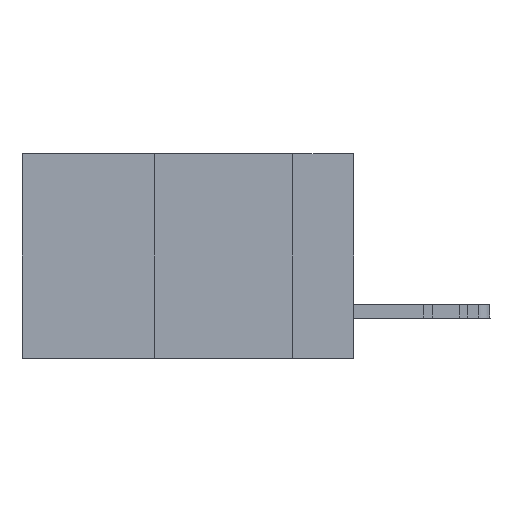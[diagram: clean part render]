
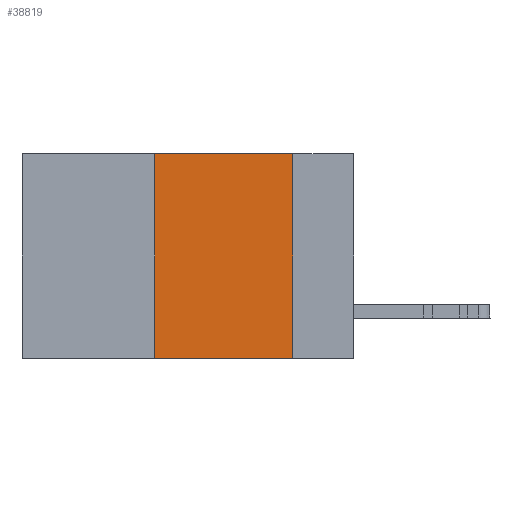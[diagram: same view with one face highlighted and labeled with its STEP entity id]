
A CAD part, left-side view. The second image highlights one B-rep face of the part: STEP entity #38819.
In plain terms, the highlighted planar face has unit normal (-1, 0, 0).
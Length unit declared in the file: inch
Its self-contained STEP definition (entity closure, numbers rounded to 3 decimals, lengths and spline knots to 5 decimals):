
#662 = CARTESIAN_POINT ( 'NONE',  ( 0., 0.36, 0. ) ) ;
#795 = VERTEX_POINT ( 'NONE', #25790 ) ;
#1541 = EDGE_CURVE ( 'NONE', #22153, #28215, #35468, .T. ) ;
#4881 = DIRECTION ( 'NONE',  ( 0., -1., 0. ) ) ;
#6494 = CARTESIAN_POINT ( 'NONE',  ( 0., 0.6, -0.37 ) ) ;
#7381 = VECTOR ( 'NONE', #44340, 39.37008 ) ;
#8488 = EDGE_CURVE ( 'NONE', #34589, #22153, #35099, .T. ) ;
#11538 = VECTOR ( 'NONE', #4881, 39.37008 ) ;
#13458 = CARTESIAN_POINT ( 'NONE',  ( 0., 0.6, 0. ) ) ;
#14044 = CARTESIAN_POINT ( 'NONE',  ( 0., 0.36, 0. ) ) ;
#14778 = DIRECTION ( 'NONE',  ( 0., 0., 1. ) ) ;
#15406 = ORIENTED_EDGE ( 'NONE', *, *, #8488, .F. ) ;
#16712 = LINE ( 'NONE', #23260, #7381 ) ;
#16812 = DIRECTION ( 'NONE',  ( 1., 0., 0. ) ) ;
#17992 = AXIS2_PLACEMENT_3D ( 'NONE', #13458, #16812, #44727 ) ;
#22118 = CARTESIAN_POINT ( 'NONE',  ( 0., 0.36, -0.37 ) ) ;
#22153 = VERTEX_POINT ( 'NONE', #662 ) ;
#23260 = CARTESIAN_POINT ( 'NONE',  ( 0., 0.11, 0. ) ) ;
#24298 = ORIENTED_EDGE ( 'NONE', *, *, #29861, .F. ) ;
#24832 = VECTOR ( 'NONE', #34191, 39.37008 ) ;
#25790 = CARTESIAN_POINT ( 'NONE',  ( 0., 0.11, -0.37 ) ) ;
#26591 = CARTESIAN_POINT ( 'NONE',  ( 0., 0.11, 0. ) ) ;
#28215 = VERTEX_POINT ( 'NONE', #26591 ) ;
#29746 = FACE_OUTER_BOUND ( 'NONE', #33715, .T. ) ;
#29861 = EDGE_CURVE ( 'NONE', #28215, #795, #16712, .T. ) ;
#31331 = ORIENTED_EDGE ( 'NONE', *, *, #1541, .F. ) ;
#33715 = EDGE_LOOP ( 'NONE', ( #24298, #31331, #15406, #44149 ) ) ;
#34191 = DIRECTION ( 'NONE',  ( 0., -1., 0. ) ) ;
#34589 = VERTEX_POINT ( 'NONE', #22118 ) ;
#35099 = LINE ( 'NONE', #14044, #43926 ) ;
#35468 = LINE ( 'NONE', #39779, #11538 ) ;
#37943 = LINE ( 'NONE', #6494, #24832 ) ;
#38147 = EDGE_CURVE ( 'NONE', #34589, #795, #37943, .T. ) ;
#38819 = ADVANCED_FACE ( 'NONE', ( #29746 ), #41371, .F. ) ;
#39779 = CARTESIAN_POINT ( 'NONE',  ( 0., 0.6, 0. ) ) ;
#41371 = PLANE ( 'NONE',  #17992 ) ;
#43926 = VECTOR ( 'NONE', #14778, 39.37008 ) ;
#44149 = ORIENTED_EDGE ( 'NONE', *, *, #38147, .T. ) ;
#44340 = DIRECTION ( 'NONE',  ( 0., 0., -1. ) ) ;
#44727 = DIRECTION ( 'NONE',  ( 0., 0., -1. ) ) ;
